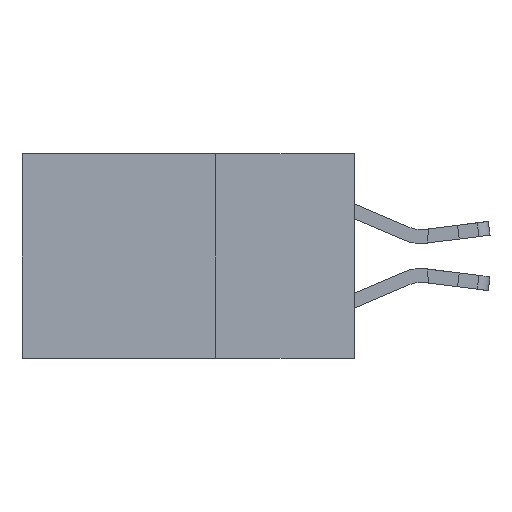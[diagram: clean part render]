
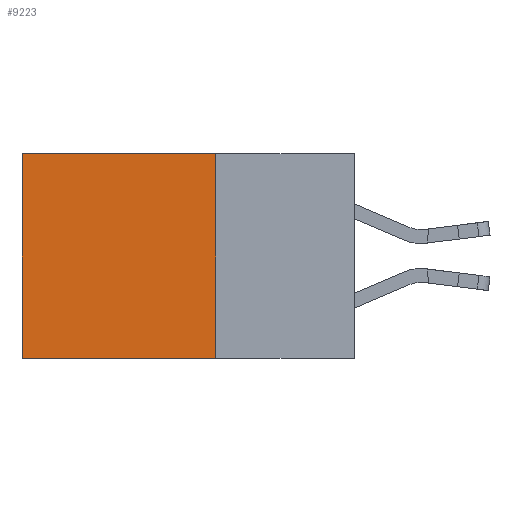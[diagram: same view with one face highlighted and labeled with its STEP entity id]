
A CAD part, left-side view. The second image highlights one B-rep face of the part: STEP entity #9223.
In plain terms, the highlighted planar face has unit normal (-1, 0, 0).
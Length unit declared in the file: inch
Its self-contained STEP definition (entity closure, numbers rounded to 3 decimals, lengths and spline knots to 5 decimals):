
#291 = ORIENTED_EDGE ( 'NONE', *, *, #11105, .F. ) ;
#617 = ORIENTED_EDGE ( 'NONE', *, *, #8590, .F. ) ;
#914 = CARTESIAN_POINT ( 'NONE',  ( 0.2615, 0.25, -0.37 ) ) ;
#1181 = LINE ( 'NONE', #4710, #3638 ) ;
#3614 = LINE ( 'NONE', #3669, #10224 ) ;
#3638 = VECTOR ( 'NONE', #8272, 39.37008 ) ;
#3651 = LINE ( 'NONE', #3823, #5991 ) ;
#3669 = CARTESIAN_POINT ( 'NONE',  ( 0.2615, 0.6, -0.37 ) ) ;
#3823 = CARTESIAN_POINT ( 'NONE',  ( 0.2615, 0.25, 0. ) ) ;
#3959 = ORIENTED_EDGE ( 'NONE', *, *, #9778, .T. ) ;
#4501 = VECTOR ( 'NONE', #5507, 39.37008 ) ;
#4710 = CARTESIAN_POINT ( 'NONE',  ( 0.2615, 0.25, -0.37 ) ) ;
#5507 = DIRECTION ( 'NONE',  ( 0., 0., -1. ) ) ;
#5554 = VERTEX_POINT ( 'NONE', #8669 ) ;
#5643 = CARTESIAN_POINT ( 'NONE',  ( 0.2615, 0.6, -0.37 ) ) ;
#5991 = VECTOR ( 'NONE', #9905, 39.37008 ) ;
#6071 = EDGE_CURVE ( 'NONE', #8689, #5554, #3651, .T. ) ;
#6289 = PLANE ( 'NONE',  #6789 ) ;
#6789 = AXIS2_PLACEMENT_3D ( 'NONE', #8826, #9045, #10717 ) ;
#6935 = ORIENTED_EDGE ( 'NONE', *, *, #6071, .T. ) ;
#7316 = DIRECTION ( 'NONE',  ( 0., 0., -1. ) ) ;
#7741 = VERTEX_POINT ( 'NONE', #914 ) ;
#8097 = VERTEX_POINT ( 'NONE', #5643 ) ;
#8267 = LINE ( 'NONE', #10795, #4501 ) ;
#8272 = DIRECTION ( 'NONE',  ( 0., 1., 0. ) ) ;
#8590 = EDGE_CURVE ( 'NONE', #7741, #8097, #1181, .T. ) ;
#8669 = CARTESIAN_POINT ( 'NONE',  ( 0.2615, 0.6, 0. ) ) ;
#8670 = EDGE_LOOP ( 'NONE', ( #3959, #617, #291, #6935 ) ) ;
#8689 = VERTEX_POINT ( 'NONE', #10450 ) ;
#8826 = CARTESIAN_POINT ( 'NONE',  ( 0.2615, 0.25, -0.37 ) ) ;
#9045 = DIRECTION ( 'NONE',  ( 1., 0., 0. ) ) ;
#9223 = ADVANCED_FACE ( 'NONE', ( #9907 ), #6289, .F. ) ;
#9778 = EDGE_CURVE ( 'NONE', #5554, #8097, #3614, .T. ) ;
#9905 = DIRECTION ( 'NONE',  ( 0., 1., 0. ) ) ;
#9907 = FACE_OUTER_BOUND ( 'NONE', #8670, .T. ) ;
#10224 = VECTOR ( 'NONE', #7316, 39.37008 ) ;
#10450 = CARTESIAN_POINT ( 'NONE',  ( 0.2615, 0.25, 0. ) ) ;
#10717 = DIRECTION ( 'NONE',  ( 0., 0., -1. ) ) ;
#10795 = CARTESIAN_POINT ( 'NONE',  ( 0.2615, 0.25, -0.37 ) ) ;
#11105 = EDGE_CURVE ( 'NONE', #8689, #7741, #8267, .T. ) ;
